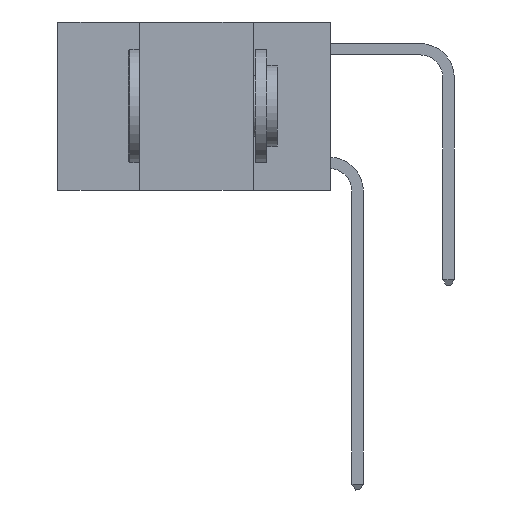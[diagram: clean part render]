
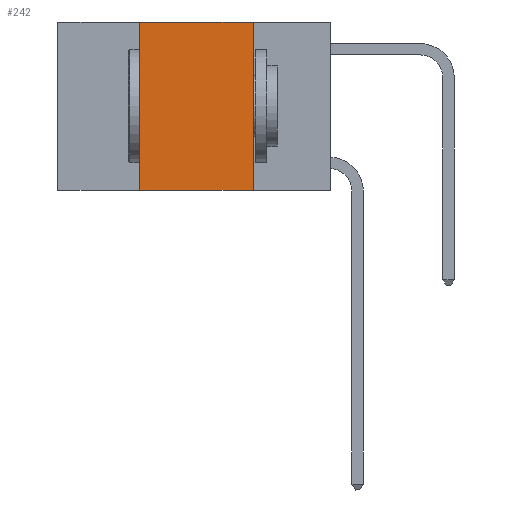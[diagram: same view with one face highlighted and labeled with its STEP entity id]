
A CAD part, left-side view. The second image highlights one B-rep face of the part: STEP entity #242.
In plain terms, the highlighted planar face has unit normal (-1, 0, 0).
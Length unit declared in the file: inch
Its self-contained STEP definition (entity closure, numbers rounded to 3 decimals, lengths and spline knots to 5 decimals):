
#242 = ADVANCED_FACE ( 'NONE', ( #5382 ), #2222, .F. ) ;
#1779 = EDGE_CURVE ( 'NONE', #6437, #8855, #18604, .T. ) ;
#2222 = PLANE ( 'NONE',  #2794 ) ;
#2452 = DIRECTION ( 'NONE',  ( 1., 0., 0. ) ) ;
#2481 = LINE ( 'NONE', #18211, #16650 ) ;
#2771 = CARTESIAN_POINT ( 'NONE',  ( 0., 0.17, 0. ) ) ;
#2794 = AXIS2_PLACEMENT_3D ( 'NONE', #11745, #2452, #13413 ) ;
#3042 = ORIENTED_EDGE ( 'NONE', *, *, #11815, .T. ) ;
#3350 = VERTEX_POINT ( 'NONE', #6040 ) ;
#4083 = CARTESIAN_POINT ( 'NONE',  ( 0., 0.17, 0. ) ) ;
#5252 = DIRECTION ( 'NONE',  ( 0., -1., 0. ) ) ;
#5382 = FACE_OUTER_BOUND ( 'NONE', #20069, .T. ) ;
#6040 = CARTESIAN_POINT ( 'NONE',  ( 0., 0.42, 0. ) ) ;
#6437 = VERTEX_POINT ( 'NONE', #4083 ) ;
#6952 = CARTESIAN_POINT ( 'NONE',  ( 0., 0.6, -0.37 ) ) ;
#7022 = VECTOR ( 'NONE', #10717, 39.37008 ) ;
#7370 = VECTOR ( 'NONE', #5252, 39.37008 ) ;
#8502 = LINE ( 'NONE', #16200, #7370 ) ;
#8855 = VERTEX_POINT ( 'NONE', #20143 ) ;
#10717 = DIRECTION ( 'NONE',  ( 0., 0., -1. ) ) ;
#11745 = CARTESIAN_POINT ( 'NONE',  ( 0., 0.6, 0. ) ) ;
#11815 = EDGE_CURVE ( 'NONE', #20108, #8855, #14863, .T. ) ;
#11978 = VECTOR ( 'NONE', #13522, 39.37008 ) ;
#12315 = ORIENTED_EDGE ( 'NONE', *, *, #1779, .F. ) ;
#13413 = DIRECTION ( 'NONE',  ( 0., 0., -1. ) ) ;
#13522 = DIRECTION ( 'NONE',  ( 0., -1., 0. ) ) ;
#13582 = EDGE_CURVE ( 'NONE', #3350, #6437, #8502, .T. ) ;
#13825 = DIRECTION ( 'NONE',  ( 0., 0., 1. ) ) ;
#14633 = ORIENTED_EDGE ( 'NONE', *, *, #13582, .F. ) ;
#14697 = ORIENTED_EDGE ( 'NONE', *, *, #19142, .F. ) ;
#14863 = LINE ( 'NONE', #6952, #11978 ) ;
#15747 = CARTESIAN_POINT ( 'NONE',  ( 0., 0.42, -0.37 ) ) ;
#16200 = CARTESIAN_POINT ( 'NONE',  ( 0., 0.6, 0. ) ) ;
#16650 = VECTOR ( 'NONE', #13825, 39.37008 ) ;
#18211 = CARTESIAN_POINT ( 'NONE',  ( 0., 0.42, 0. ) ) ;
#18604 = LINE ( 'NONE', #2771, #7022 ) ;
#19142 = EDGE_CURVE ( 'NONE', #20108, #3350, #2481, .T. ) ;
#20069 = EDGE_LOOP ( 'NONE', ( #12315, #14633, #14697, #3042 ) ) ;
#20108 = VERTEX_POINT ( 'NONE', #15747 ) ;
#20143 = CARTESIAN_POINT ( 'NONE',  ( 0., 0.17, -0.37 ) ) ;
